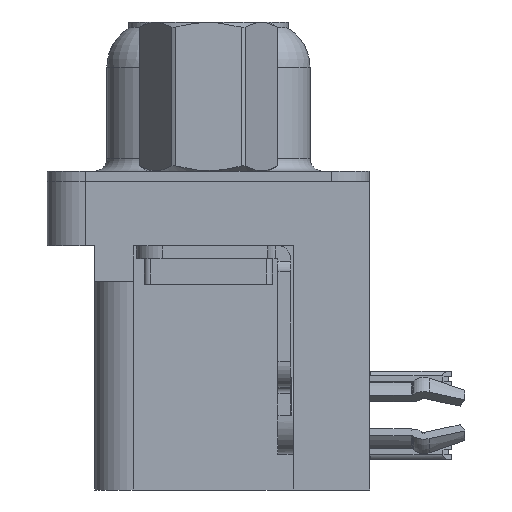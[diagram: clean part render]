
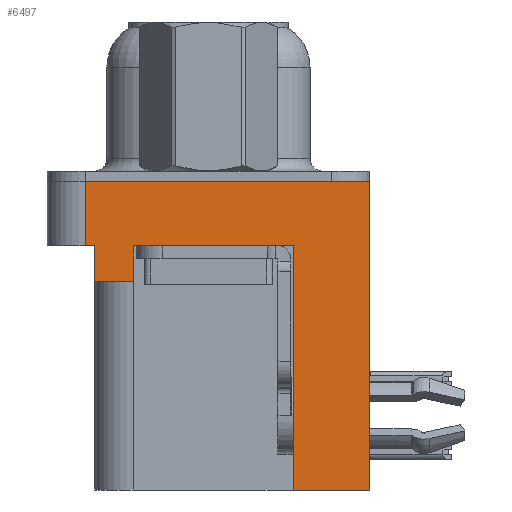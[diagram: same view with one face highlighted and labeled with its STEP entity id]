
A CAD part, left-side view. The second image highlights one B-rep face of the part: STEP entity #6497.
In plain terms, the highlighted planar face has unit normal (-1, 0, 0).
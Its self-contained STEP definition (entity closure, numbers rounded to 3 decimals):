
#133 = DIRECTION ( 'NONE',  ( 0., -1., 0. ) ) ;
#409 = VERTEX_POINT ( 'NONE', #10416 ) ;
#769 = DIRECTION ( 'NONE',  ( 0., -1., 0. ) ) ;
#1475 = CARTESIAN_POINT ( 'NONE',  ( -2.935, -6.275, -2.5 ) ) ;
#1640 = DIRECTION ( 'NONE',  ( 0., -1., 0. ) ) ;
#1641 = ORIENTED_EDGE ( 'NONE', *, *, #21778, .T. ) ;
#1767 = ORIENTED_EDGE ( 'NONE', *, *, #19786, .F. ) ;
#2252 = EDGE_CURVE ( 'NONE', #13492, #22927, #16642, .T. ) ;
#2451 = ORIENTED_EDGE ( 'NONE', *, *, #2252, .F. ) ;
#2762 = VERTEX_POINT ( 'NONE', #7269 ) ;
#2832 = CARTESIAN_POINT ( 'NONE',  ( -2.935, 2.895, -3.9 ) ) ;
#3070 = AXIS2_PLACEMENT_3D ( 'NONE', #23873, #26874, #8752 ) ;
#3265 = LINE ( 'NONE', #17973, #21487 ) ;
#3429 = DIRECTION ( 'NONE',  ( 0., 1., 0. ) ) ;
#3540 = ORIENTED_EDGE ( 'NONE', *, *, #10504, .T. ) ;
#3812 = PLANE ( 'NONE',  #3070 ) ;
#5353 = CARTESIAN_POINT ( 'NONE',  ( -2.935, -3.295, -12. ) ) ;
#6497 = ADVANCED_FACE ( 'NONE', ( #13267 ), #3812, .T. ) ;
#6542 = CARTESIAN_POINT ( 'NONE',  ( -2.935, 4.775, -2.5 ) ) ;
#7154 = VECTOR ( 'NONE', #31568, 1000. ) ;
#7269 = CARTESIAN_POINT ( 'NONE',  ( -2.935, 4.775, -2.5 ) ) ;
#7482 = CARTESIAN_POINT ( 'NONE',  ( -2.935, 4.775, 0. ) ) ;
#8752 = DIRECTION ( 'NONE',  ( 0., 0., 1. ) ) ;
#9411 = LINE ( 'NONE', #23850, #18908 ) ;
#9771 = CARTESIAN_POINT ( 'NONE',  ( -2.935, 2.895, -3.9 ) ) ;
#9917 = VECTOR ( 'NONE', #32108, 1000. ) ;
#10244 = DIRECTION ( 'NONE',  ( 0., 1., 0. ) ) ;
#10416 = CARTESIAN_POINT ( 'NONE',  ( -2.935, 4.425, -2.5 ) ) ;
#10504 = EDGE_CURVE ( 'NONE', #32259, #22927, #9411, .T. ) ;
#10812 = CARTESIAN_POINT ( 'NONE',  ( -2.935, -3.295, -12. ) ) ;
#10829 = VERTEX_POINT ( 'NONE', #21459 ) ;
#12322 = DIRECTION ( 'NONE',  ( 0., 0., 1. ) ) ;
#13085 = VERTEX_POINT ( 'NONE', #32685 ) ;
#13267 = FACE_OUTER_BOUND ( 'NONE', #22222, .T. ) ;
#13492 = VERTEX_POINT ( 'NONE', #5353 ) ;
#13824 = DIRECTION ( 'NONE',  ( 0., 0., 1. ) ) ;
#14238 = LINE ( 'NONE', #10812, #21409 ) ;
#14405 = ORIENTED_EDGE ( 'NONE', *, *, #14637, .F. ) ;
#14637 = EDGE_CURVE ( 'NONE', #10829, #13492, #14238, .T. ) ;
#14766 = VECTOR ( 'NONE', #12322, 1000. ) ;
#14918 = ORIENTED_EDGE ( 'NONE', *, *, #15036, .T. ) ;
#15036 = EDGE_CURVE ( 'NONE', #10829, #13085, #27805, .T. ) ;
#15819 = VERTEX_POINT ( 'NONE', #20434 ) ;
#16642 = LINE ( 'NONE', #27033, #9917 ) ;
#17028 = EDGE_CURVE ( 'NONE', #23629, #32259, #24614, .T. ) ;
#17362 = LINE ( 'NONE', #6542, #26492 ) ;
#17973 = CARTESIAN_POINT ( 'NONE',  ( -2.935, -6.275, -2.5 ) ) ;
#18685 = EDGE_CURVE ( 'NONE', #2762, #31825, #17362, .T. ) ;
#18794 = LINE ( 'NONE', #29291, #30004 ) ;
#18908 = VECTOR ( 'NONE', #769, 1000. ) ;
#19689 = CARTESIAN_POINT ( 'NONE',  ( -2.935, 4.425, -3.9 ) ) ;
#19786 = EDGE_CURVE ( 'NONE', #31825, #13085, #18794, .T. ) ;
#20015 = ORIENTED_EDGE ( 'NONE', *, *, #17028, .T. ) ;
#20434 = CARTESIAN_POINT ( 'NONE',  ( -2.935, 4.425, -3.9 ) ) ;
#21409 = VECTOR ( 'NONE', #3429, 1000. ) ;
#21459 = CARTESIAN_POINT ( 'NONE',  ( -2.935, -6.275, -12. ) ) ;
#21487 = VECTOR ( 'NONE', #133, 1000. ) ;
#21778 = EDGE_CURVE ( 'NONE', #2762, #409, #3265, .T. ) ;
#22089 = ORIENTED_EDGE ( 'NONE', *, *, #23246, .F. ) ;
#22222 = EDGE_LOOP ( 'NONE', ( #1767, #30351, #1641, #22665, #22089, #20015, #3540, #2451, #14405, #14918 ) ) ;
#22569 = EDGE_CURVE ( 'NONE', #15819, #409, #23100, .T. ) ;
#22665 = ORIENTED_EDGE ( 'NONE', *, *, #22569, .F. ) ;
#22749 = CARTESIAN_POINT ( 'NONE',  ( -2.935, -3.295, -2.5 ) ) ;
#22927 = VERTEX_POINT ( 'NONE', #22749 ) ;
#23100 = LINE ( 'NONE', #19689, #14766 ) ;
#23246 = EDGE_CURVE ( 'NONE', #23629, #15819, #30262, .T. ) ;
#23629 = VERTEX_POINT ( 'NONE', #9771 ) ;
#23850 = CARTESIAN_POINT ( 'NONE',  ( -2.935, -6.275, -2.5 ) ) ;
#23873 = CARTESIAN_POINT ( 'NONE',  ( -2.935, -6.275, -2.5 ) ) ;
#24614 = LINE ( 'NONE', #2832, #28997 ) ;
#26248 = VECTOR ( 'NONE', #10244, 1000. ) ;
#26492 = VECTOR ( 'NONE', #13824, 1000. ) ;
#26874 = DIRECTION ( 'NONE',  ( -1., 0., 0. ) ) ;
#27033 = CARTESIAN_POINT ( 'NONE',  ( -2.935, -3.295, -12. ) ) ;
#27805 = LINE ( 'NONE', #1475, #7154 ) ;
#28205 = DIRECTION ( 'NONE',  ( 0., 0., 1. ) ) ;
#28997 = VECTOR ( 'NONE', #28205, 1000. ) ;
#29291 = CARTESIAN_POINT ( 'NONE',  ( -2.935, -6.275, 0. ) ) ;
#30004 = VECTOR ( 'NONE', #1640, 1000. ) ;
#30262 = LINE ( 'NONE', #30372, #26248 ) ;
#30351 = ORIENTED_EDGE ( 'NONE', *, *, #18685, .F. ) ;
#30372 = CARTESIAN_POINT ( 'NONE',  ( -2.935, 4.425, -3.9 ) ) ;
#31568 = DIRECTION ( 'NONE',  ( 0., 0., 1. ) ) ;
#31645 = CARTESIAN_POINT ( 'NONE',  ( -2.935, 2.895, -2.5 ) ) ;
#31825 = VERTEX_POINT ( 'NONE', #7482 ) ;
#32108 = DIRECTION ( 'NONE',  ( 0., 0., 1. ) ) ;
#32259 = VERTEX_POINT ( 'NONE', #31645 ) ;
#32685 = CARTESIAN_POINT ( 'NONE',  ( -2.935, -6.275, 0. ) ) ;
